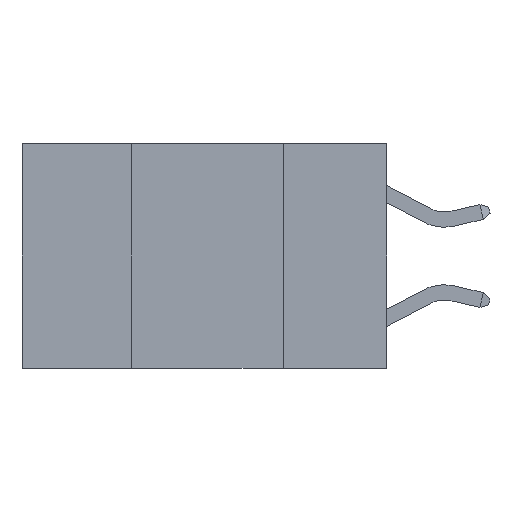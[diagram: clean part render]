
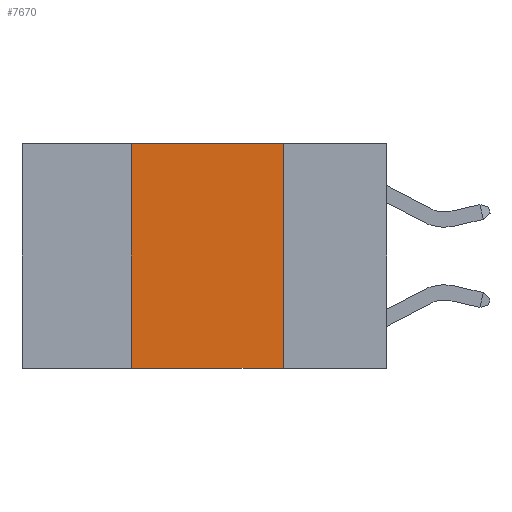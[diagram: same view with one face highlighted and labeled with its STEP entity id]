
A CAD part, left-side view. The second image highlights one B-rep face of the part: STEP entity #7670.
In plain terms, the highlighted planar face has unit normal (-1, 0, 0).
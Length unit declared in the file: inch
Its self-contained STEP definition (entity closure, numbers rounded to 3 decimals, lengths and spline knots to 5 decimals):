
#486 = LINE ( 'NONE', #10938, #954 ) ;
#954 = VECTOR ( 'NONE', #1149, 39.37008 ) ;
#1092 = VECTOR ( 'NONE', #9045, 39.37008 ) ;
#1149 = DIRECTION ( 'NONE',  ( 0., 0., 1. ) ) ;
#1582 = LINE ( 'NONE', #15517, #1092 ) ;
#1657 = VERTEX_POINT ( 'NONE', #6760 ) ;
#2771 = VERTEX_POINT ( 'NONE', #11332 ) ;
#3270 = VERTEX_POINT ( 'NONE', #12300 ) ;
#3517 = LINE ( 'NONE', #3632, #19992 ) ;
#3632 = CARTESIAN_POINT ( 'NONE',  ( 0., 0.17, 0. ) ) ;
#4946 = EDGE_CURVE ( 'NONE', #2771, #8064, #18050, .T. ) ;
#5196 = ORIENTED_EDGE ( 'NONE', *, *, #14344, .F. ) ;
#5510 = EDGE_LOOP ( 'NONE', ( #5196, #13914, #18097, #18563 ) ) ;
#6760 = CARTESIAN_POINT ( 'NONE',  ( 0., 0.17, -0.37 ) ) ;
#7670 = ADVANCED_FACE ( 'NONE', ( #9690 ), #13467, .F. ) ;
#8064 = VERTEX_POINT ( 'NONE', #17641 ) ;
#8775 = EDGE_CURVE ( 'NONE', #3270, #1657, #1582, .T. ) ;
#9045 = DIRECTION ( 'NONE',  ( 0., -1., 0. ) ) ;
#9415 = DIRECTION ( 'NONE',  ( 0., -1., 0. ) ) ;
#9690 = FACE_OUTER_BOUND ( 'NONE', #5510, .T. ) ;
#10347 = DIRECTION ( 'NONE',  ( 0., 0., -1. ) ) ;
#10938 = CARTESIAN_POINT ( 'NONE',  ( 0., 0.42, 0. ) ) ;
#11332 = CARTESIAN_POINT ( 'NONE',  ( 0., 0.42, 0. ) ) ;
#12300 = CARTESIAN_POINT ( 'NONE',  ( 0., 0.42, -0.37 ) ) ;
#13467 = PLANE ( 'NONE',  #19879 ) ;
#13472 = DIRECTION ( 'NONE',  ( 0., 0., -1. ) ) ;
#13871 = VECTOR ( 'NONE', #9415, 39.37008 ) ;
#13914 = ORIENTED_EDGE ( 'NONE', *, *, #4946, .F. ) ;
#14344 = EDGE_CURVE ( 'NONE', #8064, #1657, #3517, .T. ) ;
#15517 = CARTESIAN_POINT ( 'NONE',  ( 0., 0.6, -0.37 ) ) ;
#17147 = EDGE_CURVE ( 'NONE', #3270, #2771, #486, .T. ) ;
#17430 = CARTESIAN_POINT ( 'NONE',  ( 0., 0.6, 0. ) ) ;
#17641 = CARTESIAN_POINT ( 'NONE',  ( 0., 0.17, 0. ) ) ;
#18050 = LINE ( 'NONE', #17430, #13871 ) ;
#18097 = ORIENTED_EDGE ( 'NONE', *, *, #17147, .F. ) ;
#18256 = CARTESIAN_POINT ( 'NONE',  ( 0., 0.6, 0. ) ) ;
#18563 = ORIENTED_EDGE ( 'NONE', *, *, #8775, .T. ) ;
#19703 = DIRECTION ( 'NONE',  ( 1., 0., 0. ) ) ;
#19879 = AXIS2_PLACEMENT_3D ( 'NONE', #18256, #19703, #10347 ) ;
#19992 = VECTOR ( 'NONE', #13472, 39.37008 ) ;
